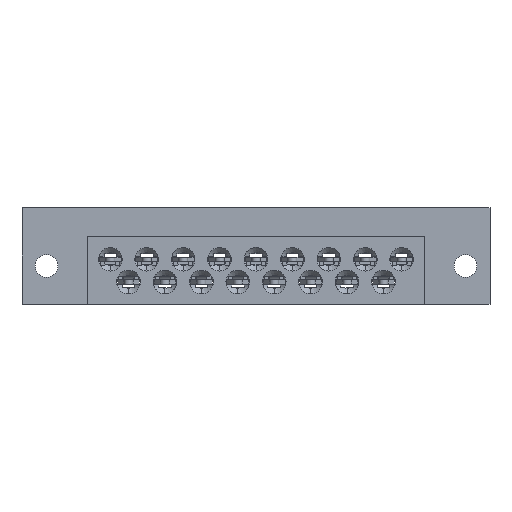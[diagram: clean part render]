
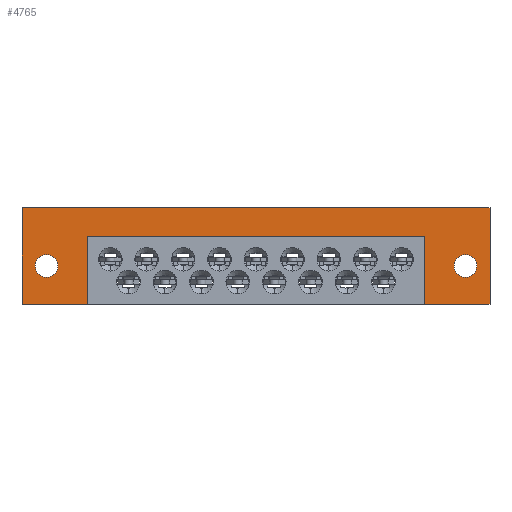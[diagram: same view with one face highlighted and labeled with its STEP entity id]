
A CAD part, front view. The second image highlights one B-rep face of the part: STEP entity #4765.
In plain terms, the highlighted planar face has unit normal (0, -1, 0).
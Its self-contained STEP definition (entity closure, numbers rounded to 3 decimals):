
#197 = VERTEX_POINT ( 'NONE', #13854 ) ;
#527 = CARTESIAN_POINT ( 'NONE',  ( 65.278, 0., 0. ) ) ;
#589 = DIRECTION ( 'NONE',  ( 0., 0., 1. ) ) ;
#655 = CIRCLE ( 'NONE', #21022, 1.587 ) ;
#798 = FACE_OUTER_BOUND ( 'NONE', #19565, .T. ) ;
#890 = PLANE ( 'NONE',  #20402 ) ;
#988 = DIRECTION ( 'NONE',  ( 0., 1., 0. ) ) ;
#1032 = CARTESIAN_POINT ( 'NONE',  ( 61.849, 0., -8.128 ) ) ;
#1122 = VERTEX_POINT ( 'NONE', #13312 ) ;
#1129 = CARTESIAN_POINT ( 'NONE',  ( 9.144, 0., -13.487 ) ) ;
#1282 = EDGE_LOOP ( 'NONE', ( #2704, #21732 ) ) ;
#1697 = VERTEX_POINT ( 'NONE', #22622 ) ;
#2265 = VERTEX_POINT ( 'NONE', #22594 ) ;
#2704 = ORIENTED_EDGE ( 'NONE', *, *, #10067, .T. ) ;
#2724 = VECTOR ( 'NONE', #15497, 1000. ) ;
#2841 = VERTEX_POINT ( 'NONE', #527 ) ;
#2882 = ORIENTED_EDGE ( 'NONE', *, *, #18768, .F. ) ;
#2887 = CIRCLE ( 'NONE', #13558, 1.588 ) ;
#3433 = DIRECTION ( 'NONE',  ( 1., 0., 0. ) ) ;
#3660 = VERTEX_POINT ( 'NONE', #9681 ) ;
#3745 = VECTOR ( 'NONE', #10830, 1000. ) ;
#4107 = EDGE_LOOP ( 'NONE', ( #16971, #22834 ) ) ;
#4274 = EDGE_CURVE ( 'NONE', #24129, #22945, #18130, .T. ) ;
#4278 = CARTESIAN_POINT ( 'NONE',  ( 3.429, 0., -9.716 ) ) ;
#4328 = DIRECTION ( 'NONE',  ( 0., 1., 0. ) ) ;
#4462 = DIRECTION ( 'NONE',  ( -1., 0., 0. ) ) ;
#4704 = DIRECTION ( 'NONE',  ( 0., 0., -1. ) ) ;
#4721 = DIRECTION ( 'NONE',  ( 0., 0., 1. ) ) ;
#4765 = ADVANCED_FACE ( 'NONE', ( #798, #20159, #14570 ), #890, .F. ) ;
#4836 = CARTESIAN_POINT ( 'NONE',  ( 9.144, 0., -3.962 ) ) ;
#5122 = VERTEX_POINT ( 'NONE', #22343 ) ;
#5246 = EDGE_CURVE ( 'NONE', #21223, #197, #8655, .T. ) ;
#5562 = CARTESIAN_POINT ( 'NONE',  ( 65.278, 0., 0. ) ) ;
#5964 = LINE ( 'NONE', #6167, #2724 ) ;
#6167 = CARTESIAN_POINT ( 'NONE',  ( 0., 0., -13.487 ) ) ;
#6277 = CARTESIAN_POINT ( 'NONE',  ( 61.849, 0., -8.128 ) ) ;
#7117 = ORIENTED_EDGE ( 'NONE', *, *, #14223, .T. ) ;
#7528 = LINE ( 'NONE', #12946, #3745 ) ;
#8060 = DIRECTION ( 'NONE',  ( 0., 0., -1. ) ) ;
#8112 = VECTOR ( 'NONE', #589, 1000. ) ;
#8311 = CARTESIAN_POINT ( 'NONE',  ( 65.278, 0., 0. ) ) ;
#8655 = CIRCLE ( 'NONE', #18689, 1.587 ) ;
#8850 = EDGE_CURVE ( 'NONE', #3660, #2265, #14657, .T. ) ;
#9295 = DIRECTION ( 'NONE',  ( -1., 0., 0. ) ) ;
#9482 = VECTOR ( 'NONE', #9295, 1000. ) ;
#9681 = CARTESIAN_POINT ( 'NONE',  ( 56.134, 0., -13.487 ) ) ;
#9981 = CARTESIAN_POINT ( 'NONE',  ( 9.144, 0., -13.488 ) ) ;
#10067 = EDGE_CURVE ( 'NONE', #12952, #22733, #2887, .T. ) ;
#10230 = ORIENTED_EDGE ( 'NONE', *, *, #8850, .T. ) ;
#10389 = EDGE_CURVE ( 'NONE', #2841, #2265, #16052, .T. ) ;
#10830 = DIRECTION ( 'NONE',  ( -1., 0., 0. ) ) ;
#11190 = DIRECTION ( 'NONE',  ( 0., 0., 1. ) ) ;
#11952 = VECTOR ( 'NONE', #8060, 1000. ) ;
#12606 = VECTOR ( 'NONE', #4704, 1000. ) ;
#12946 = CARTESIAN_POINT ( 'NONE',  ( 65.278, 0., -3.962 ) ) ;
#12952 = VERTEX_POINT ( 'NONE', #16533 ) ;
#13312 = CARTESIAN_POINT ( 'NONE',  ( 0., 0., 0. ) ) ;
#13558 = AXIS2_PLACEMENT_3D ( 'NONE', #18203, #988, #23670 ) ;
#13770 = EDGE_CURVE ( 'NONE', #197, #21223, #655, .T. ) ;
#13803 = DIRECTION ( 'NONE',  ( -1., 0., 0. ) ) ;
#13854 = CARTESIAN_POINT ( 'NONE',  ( 61.849, 0., -9.715 ) ) ;
#14125 = DIRECTION ( 'NONE',  ( 0., 1., 0. ) ) ;
#14223 = EDGE_CURVE ( 'NONE', #1697, #24129, #5964, .T. ) ;
#14488 = LINE ( 'NONE', #5562, #9482 ) ;
#14570 = FACE_BOUND ( 'NONE', #4107, .T. ) ;
#14657 = LINE ( 'NONE', #16625, #18499 ) ;
#15026 = CARTESIAN_POINT ( 'NONE',  ( 56.134, 0., -13.488 ) ) ;
#15497 = DIRECTION ( 'NONE',  ( 1., 0., 0. ) ) ;
#15938 = EDGE_CURVE ( 'NONE', #1122, #1697, #18224, .T. ) ;
#15940 = DIRECTION ( 'NONE',  ( 0., 1., 0. ) ) ;
#16052 = LINE ( 'NONE', #17523, #11952 ) ;
#16072 = ORIENTED_EDGE ( 'NONE', *, *, #19942, .F. ) ;
#16533 = CARTESIAN_POINT ( 'NONE',  ( 3.429, 0., -6.541 ) ) ;
#16625 = CARTESIAN_POINT ( 'NONE',  ( 65.278, 0., -13.487 ) ) ;
#16791 = ORIENTED_EDGE ( 'NONE', *, *, #4274, .T. ) ;
#16971 = ORIENTED_EDGE ( 'NONE', *, *, #5246, .T. ) ;
#17306 = CARTESIAN_POINT ( 'NONE',  ( 3.429, 0., -8.128 ) ) ;
#17483 = ORIENTED_EDGE ( 'NONE', *, *, #21196, .T. ) ;
#17523 = CARTESIAN_POINT ( 'NONE',  ( 65.278, 0., 0. ) ) ;
#18130 = LINE ( 'NONE', #9981, #8112 ) ;
#18144 = CARTESIAN_POINT ( 'NONE',  ( 61.849, 0., -6.541 ) ) ;
#18203 = CARTESIAN_POINT ( 'NONE',  ( 3.429, 0., -8.128 ) ) ;
#18224 = LINE ( 'NONE', #23631, #12606 ) ;
#18499 = VECTOR ( 'NONE', #3433, 1000. ) ;
#18683 = VECTOR ( 'NONE', #11190, 1000. ) ;
#18689 = AXIS2_PLACEMENT_3D ( 'NONE', #1032, #14125, #4462 ) ;
#18768 = EDGE_CURVE ( 'NONE', #5122, #22945, #7528, .T. ) ;
#18779 = AXIS2_PLACEMENT_3D ( 'NONE', #17306, #4328, #21305 ) ;
#19398 = DIRECTION ( 'NONE',  ( 0., 1., 0. ) ) ;
#19565 = EDGE_LOOP ( 'NONE', ( #21398, #7117, #16791, #2882, #16072, #10230, #22356, #17483 ) ) ;
#19942 = EDGE_CURVE ( 'NONE', #3660, #5122, #22164, .T. ) ;
#20159 = FACE_BOUND ( 'NONE', #1282, .T. ) ;
#20402 = AXIS2_PLACEMENT_3D ( 'NONE', #8311, #15940, #4721 ) ;
#21022 = AXIS2_PLACEMENT_3D ( 'NONE', #6277, #19398, #13803 ) ;
#21196 = EDGE_CURVE ( 'NONE', #2841, #1122, #14488, .T. ) ;
#21223 = VERTEX_POINT ( 'NONE', #18144 ) ;
#21305 = DIRECTION ( 'NONE',  ( -1., 0., 0. ) ) ;
#21398 = ORIENTED_EDGE ( 'NONE', *, *, #15938, .T. ) ;
#21598 = EDGE_CURVE ( 'NONE', #22733, #12952, #22816, .T. ) ;
#21732 = ORIENTED_EDGE ( 'NONE', *, *, #21598, .T. ) ;
#22164 = LINE ( 'NONE', #15026, #18683 ) ;
#22343 = CARTESIAN_POINT ( 'NONE',  ( 56.134, 0., -3.962 ) ) ;
#22356 = ORIENTED_EDGE ( 'NONE', *, *, #10389, .F. ) ;
#22594 = CARTESIAN_POINT ( 'NONE',  ( 65.278, 0., -13.487 ) ) ;
#22622 = CARTESIAN_POINT ( 'NONE',  ( 0., 0., -13.487 ) ) ;
#22733 = VERTEX_POINT ( 'NONE', #4278 ) ;
#22816 = CIRCLE ( 'NONE', #18779, 1.588 ) ;
#22834 = ORIENTED_EDGE ( 'NONE', *, *, #13770, .T. ) ;
#22945 = VERTEX_POINT ( 'NONE', #4836 ) ;
#23631 = CARTESIAN_POINT ( 'NONE',  ( 0., 0., 0. ) ) ;
#23670 = DIRECTION ( 'NONE',  ( -1., 0., 0. ) ) ;
#24129 = VERTEX_POINT ( 'NONE', #1129 ) ;
